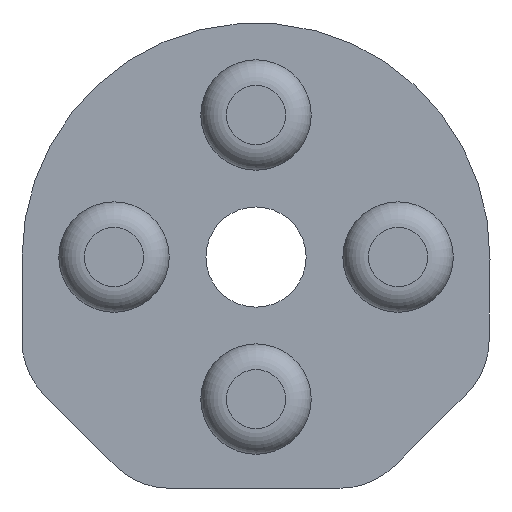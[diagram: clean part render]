
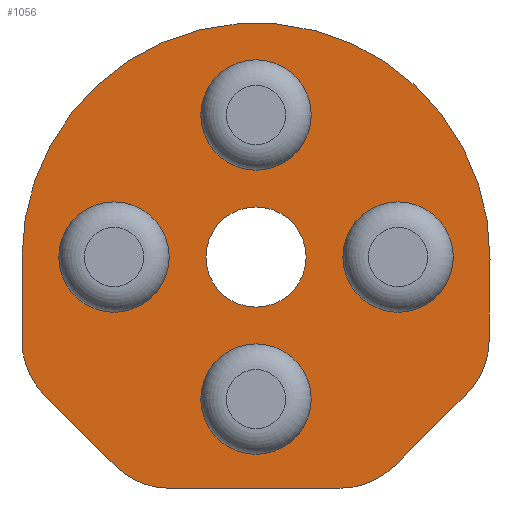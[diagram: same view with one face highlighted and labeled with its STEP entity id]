
A CAD part, front view. The second image highlights one B-rep face of the part: STEP entity #1056.
In plain terms, the highlighted planar face has unit normal (0, -1, 0).
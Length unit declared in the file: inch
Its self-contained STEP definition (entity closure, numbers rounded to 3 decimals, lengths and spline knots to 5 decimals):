
#171=CARTESIAN_POINT('',(0.215,-5.9,-0.553));
#172=VERTEX_POINT('',#171);
#173=CARTESIAN_POINT('',(0.,-5.9,-0.553));
#174=DIRECTION('',(0.0,1.0,0.0));
#175=DIRECTION('',(1.0,0.0,0.0));
#176=AXIS2_PLACEMENT_3D('',#173,#174,#175);
#177=CIRCLE('',#176,0.215);
#178=EDGE_CURVE('',#172,#172,#177,.T.);
#208=CARTESIAN_POINT('',(0.768,-5.9,0.));
#209=VERTEX_POINT('',#208);
#210=CARTESIAN_POINT('',(0.553,-5.9,0.));
#211=DIRECTION('',(0.0,1.0,0.0));
#212=DIRECTION('',(1.0,0.0,0.0));
#213=AXIS2_PLACEMENT_3D('',#210,#211,#212);
#214=CIRCLE('',#213,0.215);
#215=EDGE_CURVE('',#209,#209,#214,.T.);
#245=CARTESIAN_POINT('',(-0.338,-5.9,0.));
#246=VERTEX_POINT('',#245);
#247=CARTESIAN_POINT('',(-0.553,-5.9,0.));
#248=DIRECTION('',(0.0,1.0,0.0));
#249=DIRECTION('',(1.0,0.0,0.0));
#250=AXIS2_PLACEMENT_3D('',#247,#248,#249);
#251=CIRCLE('',#250,0.215);
#252=EDGE_CURVE('',#246,#246,#251,.T.);
#282=CARTESIAN_POINT('',(0.215,-5.9,0.553));
#283=VERTEX_POINT('',#282);
#284=CARTESIAN_POINT('',(0.0,-5.9,0.553));
#285=DIRECTION('',(0.0,1.0,0.0));
#286=DIRECTION('',(1.0,0.0,0.0));
#287=AXIS2_PLACEMENT_3D('',#284,#285,#286);
#288=CIRCLE('',#287,0.215);
#289=EDGE_CURVE('',#283,#283,#288,.T.);
#319=CARTESIAN_POINT('',(0.53764,-5.9,-0.81343));
#320=VERTEX_POINT('',#319);
#327=CARTESIAN_POINT('',(0.32682,-5.9,-0.9));
#328=VERTEX_POINT('',#327);
#329=CARTESIAN_POINT('',(0.32682,-5.9,-0.6));
#330=DIRECTION('',(0.0,1.0,0.0));
#331=DIRECTION('',(0.38,0.0,-0.925));
#332=AXIS2_PLACEMENT_3D('',#329,#330,#331);
#333=CIRCLE('',#332,0.3);
#334=EDGE_CURVE('',#320,#328,#333,.T.);
#359=CARTESIAN_POINT('',(0.8179,-5.9,-0.5366));
#360=VERTEX_POINT('',#359);
#367=CARTESIAN_POINT('',(0.8179,-5.9,-0.5366));
#368=DIRECTION('',(-0.711,0.0,-0.703));
#369=VECTOR('',#368,0.39393);
#370=LINE('',#367,#369);
#371=EDGE_CURVE('',#360,#320,#370,.T.);
#512=CARTESIAN_POINT('',(-0.33674,-5.9,-0.9));
#513=VERTEX_POINT('',#512);
#514=CARTESIAN_POINT('',(-0.54887,-5.9,-0.81213));
#515=VERTEX_POINT('',#514);
#516=CARTESIAN_POINT('',(-0.33674,-5.9,-0.6));
#517=DIRECTION('',(0.0,1.0,0.0));
#518=DIRECTION('',(-0.383,0.0,-0.924));
#519=AXIS2_PLACEMENT_3D('',#516,#517,#518);
#520=CIRCLE('',#519,0.3);
#521=EDGE_CURVE('',#513,#515,#520,.T.);
#545=CARTESIAN_POINT('',(-0.82313,-5.9,-0.53787));
#546=VERTEX_POINT('',#545);
#547=CARTESIAN_POINT('',(-0.54887,-5.9,-0.81213));
#548=DIRECTION('',(-0.707,0.0,0.707));
#549=VECTOR('',#548,0.38787);
#550=LINE('',#547,#549);
#551=EDGE_CURVE('',#515,#546,#550,.T.);
#570=CARTESIAN_POINT('',(-0.911,-5.9,-0.32574));
#571=VERTEX_POINT('',#570);
#572=CARTESIAN_POINT('',(-0.611,-5.9,-0.32574));
#573=DIRECTION('',(0.0,1.0,0.0));
#574=DIRECTION('',(-0.924,0.0,-0.383));
#575=AXIS2_PLACEMENT_3D('',#572,#573,#574);
#576=CIRCLE('',#575,0.3);
#577=EDGE_CURVE('',#546,#571,#576,.T.);
#593=CARTESIAN_POINT('',(0.90705,-5.9,-0.32686));
#594=VERTEX_POINT('',#593);
#595=CARTESIAN_POINT('',(0.60707,-5.9,-0.32317));
#596=DIRECTION('',(0.0,1.0,0.0));
#597=DIRECTION('',(0.92,0.0,-0.391));
#598=AXIS2_PLACEMENT_3D('',#595,#596,#597);
#599=CIRCLE('',#598,0.3);
#600=EDGE_CURVE('',#594,#360,#599,.T.);
#620=CARTESIAN_POINT('',(0.91093,-5.9,-0.0112));
#621=VERTEX_POINT('',#620);
#628=CARTESIAN_POINT('',(0.91093,-5.9,-0.0112));
#629=DIRECTION('',(-0.012,0.0,-1.));
#630=VECTOR('',#629,0.31568);
#631=LINE('',#628,#630);
#632=EDGE_CURVE('',#621,#594,#631,.T.);
#643=CARTESIAN_POINT('',(0.32682,-5.9,-0.9));
#644=DIRECTION('',(-1.0,0.0,0.0));
#645=VECTOR('',#644,0.66355);
#646=LINE('',#643,#645);
#647=EDGE_CURVE('',#328,#513,#646,.T.);
#967=CARTESIAN_POINT('',(-0.195,-5.9,0.0));
#968=VERTEX_POINT('',#967);
#969=CARTESIAN_POINT('',(0.0,-5.9,0.0));
#970=DIRECTION('',(0.0,1.0,0.0));
#971=DIRECTION('',(0.0,0.0,1.0));
#972=AXIS2_PLACEMENT_3D('',#969,#970,#971);
#973=CIRCLE('',#972,0.195);
#974=EDGE_CURVE('',#968,#968,#973,.T.);
#988=CARTESIAN_POINT('',(-0.911,-5.9,0.));
#989=VERTEX_POINT('',#988);
#990=CARTESIAN_POINT('',(-0.911,-5.9,-0.32574));
#991=DIRECTION('',(0.0,0.0,1.0));
#992=VECTOR('',#991,0.32574);
#993=LINE('',#990,#992);
#994=EDGE_CURVE('',#571,#989,#993,.T.);
#1011=CARTESIAN_POINT('',(0.0,-5.9,0.0));
#1012=DIRECTION('',(0.0,1.0,0.0));
#1013=DIRECTION('',(0.155,0.0,-0.988));
#1014=AXIS2_PLACEMENT_3D('',#1011,#1012,#1013);
#1015=CIRCLE('',#1014,0.911);
#1016=EDGE_CURVE('',#989,#621,#1015,.T.);
#1024=CARTESIAN_POINT('',(-0.00245,-5.9,-0.14598));
#1025=DIRECTION('',(0.0,1.0,0.0));
#1026=DIRECTION('',(0.0,0.0,1.0));
#1027=AXIS2_PLACEMENT_3D('',#1024,#1025,#1026);
#1028=PLANE('',#1027);
#1029=ORIENTED_EDGE('',*,*,#334,.F.);
#1030=ORIENTED_EDGE('',*,*,#371,.F.);
#1031=ORIENTED_EDGE('',*,*,#600,.F.);
#1032=ORIENTED_EDGE('',*,*,#632,.F.);
#1033=ORIENTED_EDGE('',*,*,#1016,.F.);
#1034=ORIENTED_EDGE('',*,*,#994,.F.);
#1035=ORIENTED_EDGE('',*,*,#577,.F.);
#1036=ORIENTED_EDGE('',*,*,#551,.F.);
#1037=ORIENTED_EDGE('',*,*,#521,.F.);
#1038=ORIENTED_EDGE('',*,*,#647,.F.);
#1039=EDGE_LOOP('',(#1029,#1030,#1031,#1032,#1033,#1034,#1035,#1036,#1037,#1038));
#1040=FACE_OUTER_BOUND('',#1039,.T.);
#1041=ORIENTED_EDGE('',*,*,#252,.T.);
#1042=EDGE_LOOP('',(#1041));
#1043=FACE_BOUND('',#1042,.T.);
#1044=ORIENTED_EDGE('',*,*,#215,.T.);
#1045=EDGE_LOOP('',(#1044));
#1046=FACE_BOUND('',#1045,.T.);
#1047=ORIENTED_EDGE('',*,*,#289,.T.);
#1048=EDGE_LOOP('',(#1047));
#1049=FACE_BOUND('',#1048,.T.);
#1050=ORIENTED_EDGE('',*,*,#178,.T.);
#1051=EDGE_LOOP('',(#1050));
#1052=FACE_BOUND('',#1051,.T.);
#1053=ORIENTED_EDGE('',*,*,#974,.T.);
#1054=EDGE_LOOP('',(#1053));
#1055=FACE_BOUND('',#1054,.T.);
#1056=ADVANCED_FACE('',(#1040,#1043,#1046,#1049,#1052,#1055),#1028,.F.);
